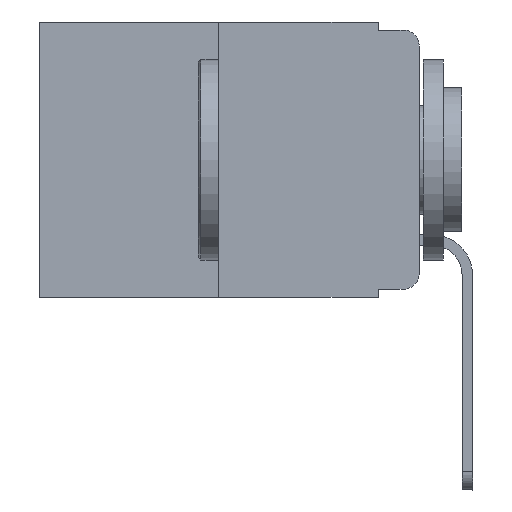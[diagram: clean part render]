
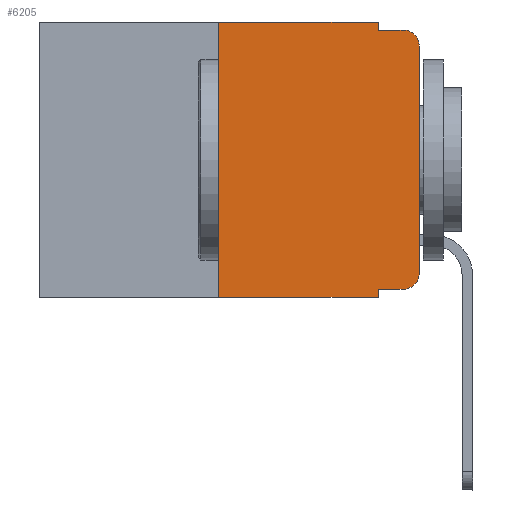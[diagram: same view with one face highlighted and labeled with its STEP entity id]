
A CAD part, left-side view. The second image highlights one B-rep face of the part: STEP entity #6205.
In plain terms, the highlighted planar face has unit normal (-1, 0, 0).
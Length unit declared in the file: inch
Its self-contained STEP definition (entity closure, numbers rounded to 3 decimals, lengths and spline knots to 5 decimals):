
#27 = LINE ( 'NONE', #3627, #8605 ) ;
#30 = FACE_OUTER_BOUND ( 'NONE', #5513, .T. ) ;
#171 = CARTESIAN_POINT ( 'NONE',  ( 0., 0.051, -0.343 ) ) ;
#203 = ORIENTED_EDGE ( 'NONE', *, *, #4551, .F. ) ;
#332 = EDGE_CURVE ( 'NONE', #9667, #4037, #7116, .T. ) ;
#411 = DIRECTION ( 'NONE',  ( -1., 0., 0. ) ) ;
#663 = ORIENTED_EDGE ( 'NONE', *, *, #4555, .F. ) ;
#750 = CARTESIAN_POINT ( 'NONE',  ( 0., 0.02, -0.333 ) ) ;
#769 = DIRECTION ( 'NONE',  ( 0., 0., -1. ) ) ;
#787 = VECTOR ( 'NONE', #5977, 39.37008 ) ;
#915 = LINE ( 'NONE', #4452, #6193 ) ;
#1020 = AXIS2_PLACEMENT_3D ( 'NONE', #4791, #4400, #2051 ) ;
#1023 = EDGE_CURVE ( 'NONE', #2795, #9036, #11088, .T. ) ;
#1292 = DIRECTION ( 'NONE',  ( 0., 0., -1. ) ) ;
#1321 = EDGE_CURVE ( 'NONE', #1568, #4468, #8137, .T. ) ;
#1568 = VERTEX_POINT ( 'NONE', #5192 ) ;
#1619 = VECTOR ( 'NONE', #1292, 39.37008 ) ;
#1690 = VECTOR ( 'NONE', #8074, 39.37008 ) ;
#1693 = CARTESIAN_POINT ( 'NONE',  ( 0., 0.02, -0.01 ) ) ;
#1867 = VECTOR ( 'NONE', #2131, 39.37008 ) ;
#1978 = CARTESIAN_POINT ( 'NONE',  ( 0., 0.051, 0. ) ) ;
#2051 = DIRECTION ( 'NONE',  ( 0., 0., -1. ) ) ;
#2131 = DIRECTION ( 'NONE',  ( 0., 0., 1. ) ) ;
#2162 = LINE ( 'NONE', #2920, #1619 ) ;
#2271 = VERTEX_POINT ( 'NONE', #171 ) ;
#2408 = EDGE_CURVE ( 'NONE', #2516, #2271, #8594, .T. ) ;
#2516 = VERTEX_POINT ( 'NONE', #9932 ) ;
#2659 = ORIENTED_EDGE ( 'NONE', *, *, #332, .F. ) ;
#2788 = DIRECTION ( 'NONE',  ( -1., 0., 0. ) ) ;
#2795 = VERTEX_POINT ( 'NONE', #9666 ) ;
#2920 = CARTESIAN_POINT ( 'NONE',  ( 0., 0.051, 0. ) ) ;
#3220 = DIRECTION ( 'NONE',  ( 0., -1., 0. ) ) ;
#3515 = CARTESIAN_POINT ( 'NONE',  ( 0., 0.051, -0.333 ) ) ;
#3627 = CARTESIAN_POINT ( 'NONE',  ( 0., 0.473, 0. ) ) ;
#3693 = VECTOR ( 'NONE', #3220, 39.37008 ) ;
#4037 = VERTEX_POINT ( 'NONE', #1693 ) ;
#4150 = ORIENTED_EDGE ( 'NONE', *, *, #10389, .T. ) ;
#4400 = DIRECTION ( 'NONE',  ( 1., 0., 0. ) ) ;
#4452 = CARTESIAN_POINT ( 'NONE',  ( 0., 0.25, 0. ) ) ;
#4468 = VERTEX_POINT ( 'NONE', #750 ) ;
#4551 = EDGE_CURVE ( 'NONE', #2516, #4699, #915, .T. ) ;
#4555 = EDGE_CURVE ( 'NONE', #4699, #6708, #27, .T. ) ;
#4699 = VERTEX_POINT ( 'NONE', #9186 ) ;
#4791 = CARTESIAN_POINT ( 'NONE',  ( 0., 0.473, 0. ) ) ;
#5063 = ORIENTED_EDGE ( 'NONE', *, *, #8994, .T. ) ;
#5101 = ORIENTED_EDGE ( 'NONE', *, *, #1023, .T. ) ;
#5192 = CARTESIAN_POINT ( 'NONE',  ( 0., 0.051, -0.333 ) ) ;
#5269 = CARTESIAN_POINT ( 'NONE',  ( 0., 0.473, -0.343 ) ) ;
#5364 = VECTOR ( 'NONE', #11244, 39.37008 ) ;
#5513 = EDGE_LOOP ( 'NONE', ( #5101, #4150, #2659, #6727, #663, #203, #7242, #11278, #10700, #5063 ) ) ;
#5977 = DIRECTION ( 'NONE',  ( 0., -1., 0. ) ) ;
#6193 = VECTOR ( 'NONE', #8017, 39.37008 ) ;
#6205 = ADVANCED_FACE ( 'NONE', ( #30 ), #9290, .F. ) ;
#6574 = CARTESIAN_POINT ( 'NONE',  ( 0., 0., 0. ) ) ;
#6708 = VERTEX_POINT ( 'NONE', #1978 ) ;
#6727 = ORIENTED_EDGE ( 'NONE', *, *, #8704, .F. ) ;
#7063 = CARTESIAN_POINT ( 'NONE',  ( 0., 0., -0.03 ) ) ;
#7116 = LINE ( 'NONE', #11184, #3693 ) ;
#7242 = ORIENTED_EDGE ( 'NONE', *, *, #2408, .T. ) ;
#7509 = DIRECTION ( 'NONE',  ( 0., -1., 0. ) ) ;
#7894 = LINE ( 'NONE', #8579, #5364 ) ;
#8017 = DIRECTION ( 'NONE',  ( 0., 0., 1. ) ) ;
#8074 = DIRECTION ( 'NONE',  ( 0., -1., 0. ) ) ;
#8137 = LINE ( 'NONE', #3515, #1690 ) ;
#8274 = DIRECTION ( 'NONE',  ( 0., 0., -1. ) ) ;
#8579 = CARTESIAN_POINT ( 'NONE',  ( 0., 0.051, 0. ) ) ;
#8594 = LINE ( 'NONE', #5269, #787 ) ;
#8605 = VECTOR ( 'NONE', #7509, 39.37008 ) ;
#8704 = EDGE_CURVE ( 'NONE', #6708, #9667, #2162, .T. ) ;
#8994 = EDGE_CURVE ( 'NONE', #4468, #2795, #11092, .T. ) ;
#9036 = VERTEX_POINT ( 'NONE', #7063 ) ;
#9186 = CARTESIAN_POINT ( 'NONE',  ( 0., 0.25, 0. ) ) ;
#9290 = PLANE ( 'NONE',  #1020 ) ;
#9581 = CARTESIAN_POINT ( 'NONE',  ( 0., 0.051, -0.01 ) ) ;
#9660 = EDGE_CURVE ( 'NONE', #1568, #2271, #7894, .T. ) ;
#9666 = CARTESIAN_POINT ( 'NONE',  ( 0., 0., -0.313 ) ) ;
#9667 = VERTEX_POINT ( 'NONE', #9581 ) ;
#9805 = AXIS2_PLACEMENT_3D ( 'NONE', #9841, #2788, #769 ) ;
#9841 = CARTESIAN_POINT ( 'NONE',  ( 0., 0.02, -0.313 ) ) ;
#9932 = CARTESIAN_POINT ( 'NONE',  ( 0., 0.25, -0.343 ) ) ;
#10371 = CIRCLE ( 'NONE', #10552, 0.02 ) ;
#10389 = EDGE_CURVE ( 'NONE', #9036, #4037, #10371, .T. ) ;
#10552 = AXIS2_PLACEMENT_3D ( 'NONE', #10981, #411, #8274 ) ;
#10700 = ORIENTED_EDGE ( 'NONE', *, *, #1321, .T. ) ;
#10981 = CARTESIAN_POINT ( 'NONE',  ( 0., 0.02, -0.03 ) ) ;
#11088 = LINE ( 'NONE', #6574, #1867 ) ;
#11092 = CIRCLE ( 'NONE', #9805, 0.02 ) ;
#11184 = CARTESIAN_POINT ( 'NONE',  ( 0., 0.051, -0.01 ) ) ;
#11244 = DIRECTION ( 'NONE',  ( 0., 0., -1. ) ) ;
#11278 = ORIENTED_EDGE ( 'NONE', *, *, #9660, .F. ) ;
